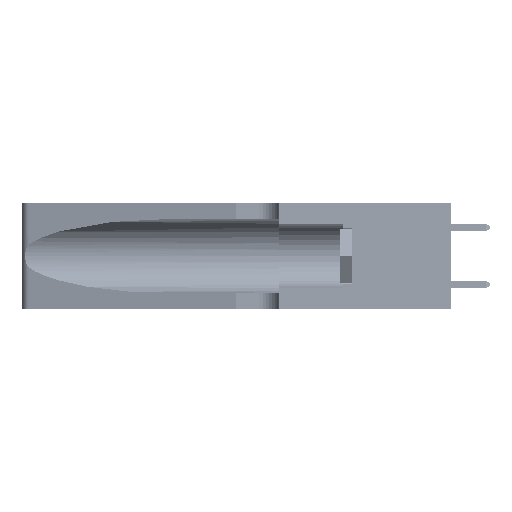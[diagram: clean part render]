
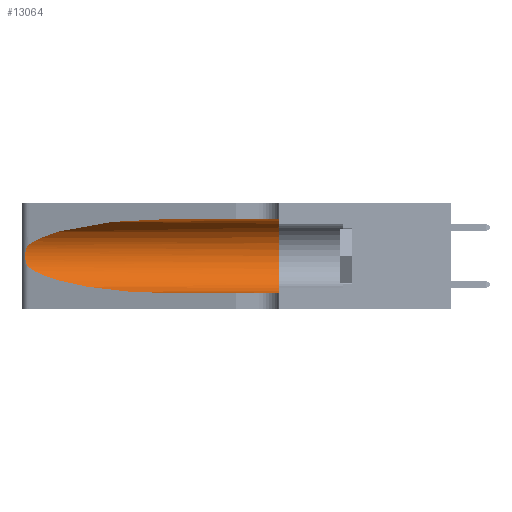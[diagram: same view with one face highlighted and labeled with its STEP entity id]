
A CAD part, left-side view. The second image highlights one B-rep face of the part: STEP entity #13064.
In plain terms, the highlighted cylindrical face has radius 3.308 mm (diameter 6.617 mm), a partial arc.
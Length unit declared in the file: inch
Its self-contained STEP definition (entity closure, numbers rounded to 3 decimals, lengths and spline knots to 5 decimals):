
#442 = CARTESIAN_POINT ( 'NONE',  ( 0.25787, 1.23484, 0.2124 ) ) ;
#613 = ORIENTED_EDGE ( 'NONE', *, *, #42870, .F. ) ;
#1076 = CARTESIAN_POINT ( 'NONE',  ( 0.1305, 0.72297, 0.05475 ) ) ;
#2151 = CARTESIAN_POINT ( 'NONE',  ( 0.1305, 0.35, 0.185 ) ) ;
#2651 = CIRCLE ( 'NONE', #16162, 0.13025 ) ;
#2781 = CYLINDRICAL_SURFACE ( 'NONE', #8144, 0.13025 ) ;
#4075 = VECTOR ( 'NONE', #23808, 39.37008 ) ;
#4170 = EDGE_LOOP ( 'NONE', ( #37199, #25497, #21394, #38236, #613, #9239 ) ) ;
#4269 = CARTESIAN_POINT ( 'NONE',  ( 0.26018, 1.23835, 0.19895 ) ) ;
#4871 = CARTESIAN_POINT ( 'NONE',  ( 0.2373, 1.15595, 0.28018 ) ) ;
#5001 =( BOUNDED_CURVE ( )  B_SPLINE_CURVE ( 3, ( #27715, #43034, #24046, #1076 ),
 .UNSPECIFIED., .F., .T. ) 
 B_SPLINE_CURVE_WITH_KNOTS ( ( 4, 4 ),
 ( 3.44316, 4.71239 ),
 .UNSPECIFIED. ) 
 CURVE ( )  GEOMETRIC_REPRESENTATION_ITEM ( )  RATIONAL_B_SPLINE_CURVE ( ( 1., 0.87, 0.87, 1. ) ) 
 REPRESENTATION_ITEM ( '' )  );
#6000 = DIRECTION ( 'NONE',  ( 0., 0., 1. ) ) ;
#8116 = CARTESIAN_POINT ( 'NONE',  ( 0.26075, 1.23896, 0.178 ) ) ;
#8144 = AXIS2_PLACEMENT_3D ( 'NONE', #33025, #29224, #10071 ) ;
#9239 = ORIENTED_EDGE ( 'NONE', *, *, #12127, .F. ) ;
#10071 = DIRECTION ( 'NONE',  ( 0., 0., -1. ) ) ;
#10862 = VERTEX_POINT ( 'NONE', #43733 ) ;
#11968 = CARTESIAN_POINT ( 'NONE',  ( 0.1305, 0.35, 0.31525 ) ) ;
#11982 = CARTESIAN_POINT ( 'NONE',  ( 0.25856, 1.23593, 0.16098 ) ) ;
#12127 = EDGE_CURVE ( 'NONE', #23336, #38703, #35803, .T. ) ;
#13064 = ADVANCED_FACE ( 'NONE', ( #23195 ), #2781, .F. ) ;
#13779 = EDGE_CURVE ( 'NONE', #46651, #35988, #41091, .T. ) ;
#15680 = CARTESIAN_POINT ( 'NONE',  ( 0.25555, 1.22994, 0.2215 ) ) ;
#15847 = CARTESIAN_POINT ( 'NONE',  ( 0.25639, 1.23186, 0.15144 ) ) ;
#16162 = AXIS2_PLACEMENT_3D ( 'NONE', #2151, #28991, #6000 ) ;
#16270 = CARTESIAN_POINT ( 'NONE',  ( 0.18966, 0.96281, 0.31525 ) ) ;
#16615 = CARTESIAN_POINT ( 'NONE',  ( 0.25487, 1.22718, 0.14631 ) ) ;
#17906 = CARTESIAN_POINT ( 'NONE',  ( 0.1305, 1.61858, 0.05475 ) ) ;
#19699 = CARTESIAN_POINT ( 'NONE',  ( 0.25487, 1.22718, 0.14631 ) ) ;
#20098 = CARTESIAN_POINT ( 'NONE',  ( 0.1305, 1.61858, 0.31525 ) ) ;
#20109 = CARTESIAN_POINT ( 'NONE',  ( 0.1305, 0.72297, 0.31525 ) ) ;
#21394 = ORIENTED_EDGE ( 'NONE', *, *, #45013, .T. ) ;
#21773 = DIRECTION ( 'NONE',  ( 0., -1., 0. ) ) ;
#22412 = VERTEX_POINT ( 'NONE', #16615 ) ;
#23195 = FACE_OUTER_BOUND ( 'NONE', #4170, .T. ) ;
#23336 = VERTEX_POINT ( 'NONE', #37099 ) ;
#23403 = CARTESIAN_POINT ( 'NONE',  ( 0.25639, 1.23184, 0.21858 ) ) ;
#23453 = CARTESIAN_POINT ( 'NONE',  ( 0.1305, 0.35, 0.05475 ) ) ;
#23587 = EDGE_CURVE ( 'NONE', #10862, #22412, #47885, .T. ) ;
#23808 = DIRECTION ( 'NONE',  ( 0., -1., 0. ) ) ;
#24046 = CARTESIAN_POINT ( 'NONE',  ( 0.18966, 0.96281, 0.05475 ) ) ;
#25497 = ORIENTED_EDGE ( 'NONE', *, *, #23587, .T. ) ;
#27234 = CARTESIAN_POINT ( 'NONE',  ( 0.25854, 1.2359, 0.20912 ) ) ;
#27715 = CARTESIAN_POINT ( 'NONE',  ( 0.25487, 1.22718, 0.14631 ) ) ;
#28991 = DIRECTION ( 'NONE',  ( 0., 1., 0. ) ) ;
#29224 = DIRECTION ( 'NONE',  ( 0., -1., 0. ) ) ;
#31096 = CARTESIAN_POINT ( 'NONE',  ( 0.26075, 1.23896, 0.19203 ) ) ;
#31675 = CARTESIAN_POINT ( 'NONE',  ( 0.25487, 1.22718, 0.22369 ) ) ;
#33025 = CARTESIAN_POINT ( 'NONE',  ( 0.1305, 1.61858, 0.185 ) ) ;
#34894 = CARTESIAN_POINT ( 'NONE',  ( 0.26017, 1.23833, 0.17102 ) ) ;
#35803 = LINE ( 'NONE', #20098, #4075 ) ;
#35988 = VERTEX_POINT ( 'NONE', #23453 ) ;
#36909 =( BOUNDED_CURVE ( )  B_SPLINE_CURVE ( 3, ( #20109, #16270, #4871, #31675 ),
 .UNSPECIFIED., .F., .T. ) 
 B_SPLINE_CURVE_WITH_KNOTS ( ( 4, 4 ),
 ( 1.5708, 2.84003 ),
 .UNSPECIFIED. ) 
 CURVE ( )  GEOMETRIC_REPRESENTATION_ITEM ( )  RATIONAL_B_SPLINE_CURVE ( ( 1., 0.87, 0.87, 1. ) ) 
 REPRESENTATION_ITEM ( '' )  );
#37099 = CARTESIAN_POINT ( 'NONE',  ( 0.1305, 0.72297, 0.31525 ) ) ;
#37199 = ORIENTED_EDGE ( 'NONE', *, *, #45724, .T. ) ;
#38236 = ORIENTED_EDGE ( 'NONE', *, *, #13779, .T. ) ;
#38703 = VERTEX_POINT ( 'NONE', #11968 ) ;
#38735 = CARTESIAN_POINT ( 'NONE',  ( 0.25789, 1.23486, 0.15765 ) ) ;
#39896 = VECTOR ( 'NONE', #21773, 39.37008 ) ;
#41091 = LINE ( 'NONE', #17906, #39896 ) ;
#42402 = CARTESIAN_POINT ( 'NONE',  ( 0.25487, 1.22718, 0.22369 ) ) ;
#42559 = CARTESIAN_POINT ( 'NONE',  ( 0.25555, 1.22993, 0.14849 ) ) ;
#42870 = EDGE_CURVE ( 'NONE', #38703, #35988, #2651, .T. ) ;
#43034 = CARTESIAN_POINT ( 'NONE',  ( 0.2373, 1.15595, 0.08982 ) ) ;
#43733 = CARTESIAN_POINT ( 'NONE',  ( 0.25487, 1.22718, 0.22369 ) ) ;
#44749 = CARTESIAN_POINT ( 'NONE',  ( 0.1305, 0.72297, 0.05475 ) ) ;
#45013 = EDGE_CURVE ( 'NONE', #22412, #46651, #5001, .T. ) ;
#45724 = EDGE_CURVE ( 'NONE', #23336, #10862, #36909, .T. ) ;
#46651 = VERTEX_POINT ( 'NONE', #44749 ) ;
#47885 = B_SPLINE_CURVE_WITH_KNOTS ( 'NONE', 3,
 ( #42402, #15680, #23403, #442, #27234, #4269, #31096, #8116, #34894, #11982, #38735, #15847, #42559, #19699 ),
 .UNSPECIFIED., .F., .F.,
 ( 4, 2, 2, 2, 2, 2, 4 ),
 ( 0., 0.00027, 0.00053, 0.00107, 0.0016, 0.00187, 0.00214 ),
 .UNSPECIFIED. ) ;
